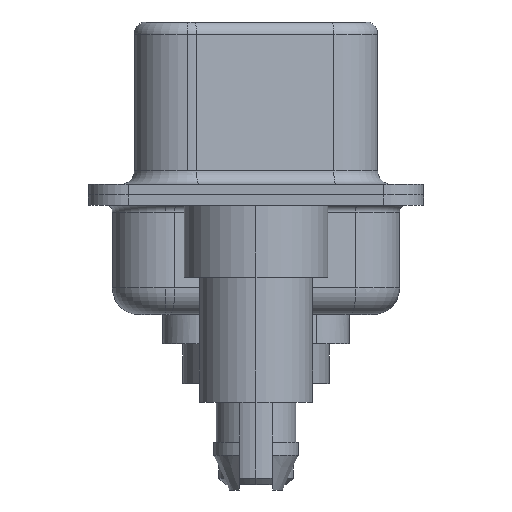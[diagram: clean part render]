
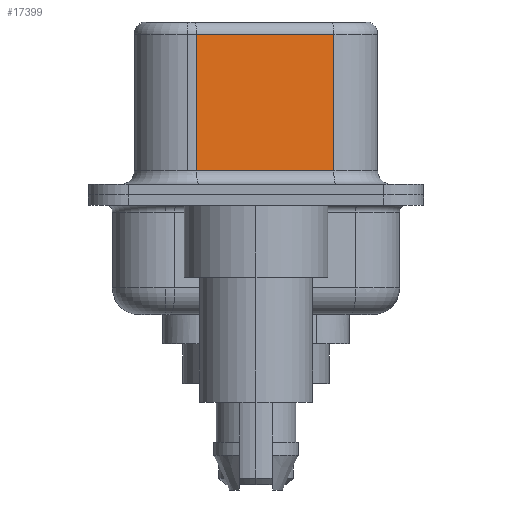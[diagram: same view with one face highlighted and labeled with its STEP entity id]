
A CAD part, left-side view. The second image highlights one B-rep face of the part: STEP entity #17399.
In plain terms, the highlighted planar face has unit normal (-0.985, -0.174, 0).
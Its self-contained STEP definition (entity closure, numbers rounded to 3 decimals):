
#1041 = LINE ( 'NONE', #10693, #5087 ) ;
#1382 = ORIENTED_EDGE ( 'NONE', *, *, #17790, .T. ) ;
#2514 = EDGE_CURVE ( 'NONE', #18894, #18066, #14901, .T. ) ;
#3386 = VERTEX_POINT ( 'NONE', #14367 ) ;
#3470 = CARTESIAN_POINT ( 'NONE',  ( 3.67, 2.233, 6.02 ) ) ;
#3624 = LINE ( 'NONE', #8284, #15011 ) ;
#5087 = VECTOR ( 'NONE', #16609, 1000. ) ;
#5652 = ORIENTED_EDGE ( 'NONE', *, *, #11731, .F. ) ;
#5824 = CARTESIAN_POINT ( 'NONE',  ( 3.67, 2.233, 6.52 ) ) ;
#6044 = LINE ( 'NONE', #5824, #9965 ) ;
#6406 = CARTESIAN_POINT ( 'NONE',  ( 4.58, -2.927, 6.52 ) ) ;
#6561 = VECTOR ( 'NONE', #19194, 1000. ) ;
#7357 = DIRECTION ( 'NONE',  ( 0., 0., -1. ) ) ;
#7905 = DIRECTION ( 'NONE',  ( 0.985, 0.174, 0. ) ) ;
#8284 = CARTESIAN_POINT ( 'NONE',  ( 4.58, -2.927, 6.52 ) ) ;
#9965 = VECTOR ( 'NONE', #7357, 1000. ) ;
#10604 = VERTEX_POINT ( 'NONE', #15453 ) ;
#10693 = CARTESIAN_POINT ( 'NONE',  ( 4.58, -2.927, 0.9 ) ) ;
#11731 = EDGE_CURVE ( 'NONE', #18894, #10604, #3624, .T. ) ;
#12703 = DIRECTION ( 'NONE',  ( 0., 0., -1. ) ) ;
#12905 = ORIENTED_EDGE ( 'NONE', *, *, #17955, .T. ) ;
#13292 = FACE_OUTER_BOUND ( 'NONE', #17310, .T. ) ;
#14367 = CARTESIAN_POINT ( 'NONE',  ( 3.67, 2.233, 0.9 ) ) ;
#14901 = LINE ( 'NONE', #18548, #6561 ) ;
#14920 = CARTESIAN_POINT ( 'NONE',  ( 4.58, -2.927, 6.02 ) ) ;
#15011 = VECTOR ( 'NONE', #12703, 1000. ) ;
#15037 = AXIS2_PLACEMENT_3D ( 'NONE', #6406, #7905, #18181 ) ;
#15255 = PLANE ( 'NONE',  #15037 ) ;
#15453 = CARTESIAN_POINT ( 'NONE',  ( 4.58, -2.927, 0.9 ) ) ;
#16609 = DIRECTION ( 'NONE',  ( 0.174, -0.985, 0. ) ) ;
#17310 = EDGE_LOOP ( 'NONE', ( #5652, #19072, #1382, #12905 ) ) ;
#17399 = ADVANCED_FACE ( 'NONE', ( #13292 ), #15255, .F. ) ;
#17790 = EDGE_CURVE ( 'NONE', #18066, #3386, #6044, .T. ) ;
#17955 = EDGE_CURVE ( 'NONE', #3386, #10604, #1041, .T. ) ;
#18066 = VERTEX_POINT ( 'NONE', #3470 ) ;
#18181 = DIRECTION ( 'NONE',  ( -0.174, 0.985, 0. ) ) ;
#18548 = CARTESIAN_POINT ( 'NONE',  ( 4.58, -2.927, 6.02 ) ) ;
#18894 = VERTEX_POINT ( 'NONE', #14920 ) ;
#19072 = ORIENTED_EDGE ( 'NONE', *, *, #2514, .T. ) ;
#19194 = DIRECTION ( 'NONE',  ( -0.174, 0.985, 0. ) ) ;
